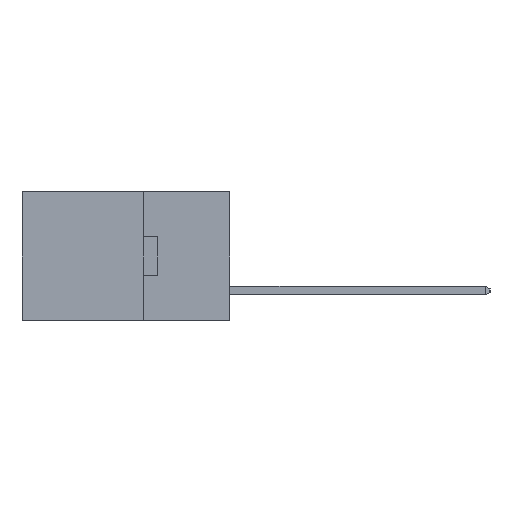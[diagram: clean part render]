
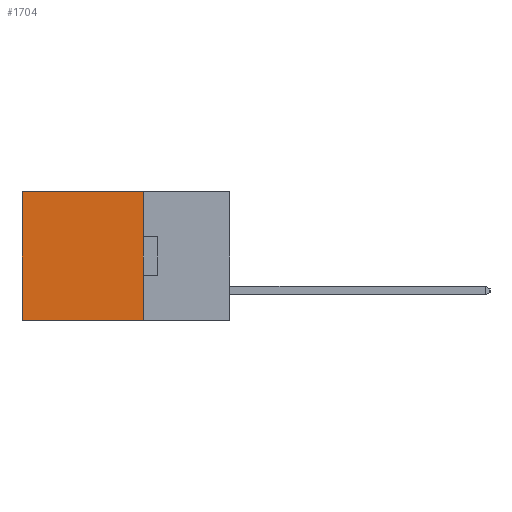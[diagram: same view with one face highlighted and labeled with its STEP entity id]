
A CAD part, left-side view. The second image highlights one B-rep face of the part: STEP entity #1704.
In plain terms, the highlighted planar face has unit normal (-1, 0, 0).
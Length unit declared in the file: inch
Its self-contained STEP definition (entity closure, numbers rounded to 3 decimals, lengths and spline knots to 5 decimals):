
#186 = EDGE_CURVE ( 'NONE', #16323, #8354, #15228, .T. ) ;
#651 = DIRECTION ( 'NONE',  ( 0., 0., -1. ) ) ;
#739 = DIRECTION ( 'NONE',  ( 1., 0., 0. ) ) ;
#860 = CARTESIAN_POINT ( 'NONE',  ( 0.2615, 0.25, -0.37 ) ) ;
#1268 = PLANE ( 'NONE',  #23774 ) ;
#1363 = CARTESIAN_POINT ( 'NONE',  ( 0.2615, 0.6, 0. ) ) ;
#1704 = ADVANCED_FACE ( 'NONE', ( #26570 ), #1268, .F. ) ;
#4531 = ORIENTED_EDGE ( 'NONE', *, *, #15835, .F. ) ;
#4864 = VECTOR ( 'NONE', #11764, 39.37008 ) ;
#5192 = CARTESIAN_POINT ( 'NONE',  ( 0.2615, 0.25, 0. ) ) ;
#6126 = ORIENTED_EDGE ( 'NONE', *, *, #9195, .F. ) ;
#6413 = LINE ( 'NONE', #12825, #22144 ) ;
#7305 = DIRECTION ( 'NONE',  ( 0., 1., 0. ) ) ;
#8354 = VERTEX_POINT ( 'NONE', #22241 ) ;
#8374 = ORIENTED_EDGE ( 'NONE', *, *, #186, .T. ) ;
#8683 = LINE ( 'NONE', #12844, #13506 ) ;
#9195 = EDGE_CURVE ( 'NONE', #19478, #8354, #6413, .T. ) ;
#9398 = CARTESIAN_POINT ( 'NONE',  ( 0.2615, 0.25, -0.37 ) ) ;
#11539 = CARTESIAN_POINT ( 'NONE',  ( 0.2615, 0.6, -0.37 ) ) ;
#11764 = DIRECTION ( 'NONE',  ( 0., 0., -1. ) ) ;
#12044 = EDGE_LOOP ( 'NONE', ( #8374, #6126, #4531, #18567 ) ) ;
#12825 = CARTESIAN_POINT ( 'NONE',  ( 0.2615, 0.25, -0.37 ) ) ;
#12844 = CARTESIAN_POINT ( 'NONE',  ( 0.2615, 0.25, -0.37 ) ) ;
#13506 = VECTOR ( 'NONE', #25040, 39.37008 ) ;
#14544 = VERTEX_POINT ( 'NONE', #16788 ) ;
#14724 = LINE ( 'NONE', #5192, #24904 ) ;
#15228 = LINE ( 'NONE', #11539, #4864 ) ;
#15835 = EDGE_CURVE ( 'NONE', #14544, #19478, #8683, .T. ) ;
#16323 = VERTEX_POINT ( 'NONE', #1363 ) ;
#16788 = CARTESIAN_POINT ( 'NONE',  ( 0.2615, 0.25, 0. ) ) ;
#16973 = DIRECTION ( 'NONE',  ( 0., 1., 0. ) ) ;
#18567 = ORIENTED_EDGE ( 'NONE', *, *, #23032, .T. ) ;
#19478 = VERTEX_POINT ( 'NONE', #9398 ) ;
#22144 = VECTOR ( 'NONE', #16973, 39.37008 ) ;
#22241 = CARTESIAN_POINT ( 'NONE',  ( 0.2615, 0.6, -0.37 ) ) ;
#23032 = EDGE_CURVE ( 'NONE', #14544, #16323, #14724, .T. ) ;
#23774 = AXIS2_PLACEMENT_3D ( 'NONE', #860, #739, #651 ) ;
#24904 = VECTOR ( 'NONE', #7305, 39.37008 ) ;
#25040 = DIRECTION ( 'NONE',  ( 0., 0., -1. ) ) ;
#26570 = FACE_OUTER_BOUND ( 'NONE', #12044, .T. ) ;
